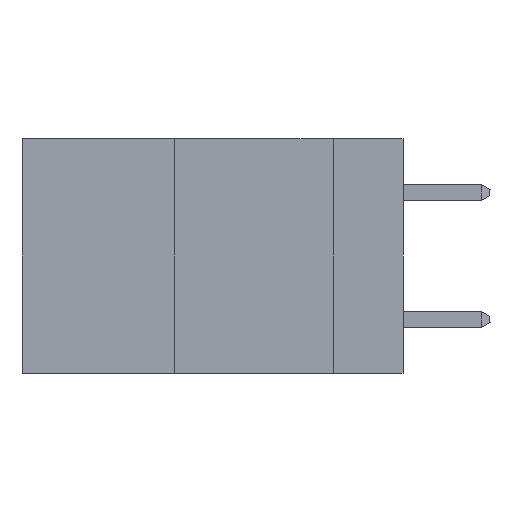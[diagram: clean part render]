
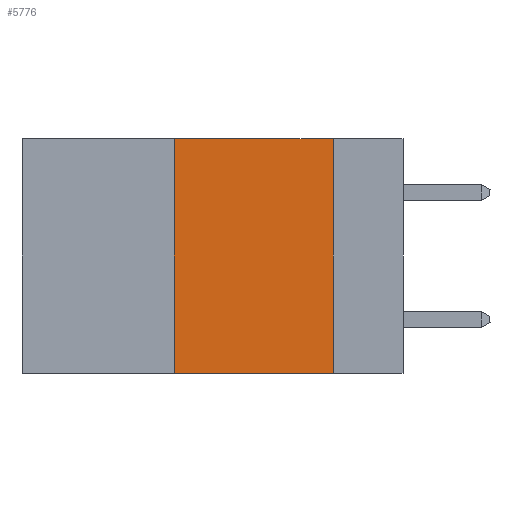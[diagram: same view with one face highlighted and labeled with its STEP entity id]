
A CAD part, left-side view. The second image highlights one B-rep face of the part: STEP entity #5776.
In plain terms, the highlighted planar face has unit normal (-1, 0, 0).
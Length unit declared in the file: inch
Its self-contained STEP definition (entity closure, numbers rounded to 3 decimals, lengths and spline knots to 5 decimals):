
#298 = DIRECTION ( 'NONE',  ( 0., 0., -1. ) ) ;
#560 = VECTOR ( 'NONE', #26376, 39.37008 ) ;
#3528 = CARTESIAN_POINT ( 'NONE',  ( 0., 0.11, 0. ) ) ;
#5776 = ADVANCED_FACE ( 'NONE', ( #25094 ), #15603, .F. ) ;
#8339 = VERTEX_POINT ( 'NONE', #15843 ) ;
#8670 = LINE ( 'NONE', #34059, #17646 ) ;
#11580 = VECTOR ( 'NONE', #31246, 39.37008 ) ;
#11921 = CARTESIAN_POINT ( 'NONE',  ( 0., 0.11, 0. ) ) ;
#13233 = VECTOR ( 'NONE', #298, 39.37008 ) ;
#13871 = DIRECTION ( 'NONE',  ( 0., -1., 0. ) ) ;
#14397 = LINE ( 'NONE', #29242, #560 ) ;
#15320 = ORIENTED_EDGE ( 'NONE', *, *, #20392, .T. ) ;
#15603 = PLANE ( 'NONE',  #24603 ) ;
#15730 = ORIENTED_EDGE ( 'NONE', *, *, #36065, .F. ) ;
#15843 = CARTESIAN_POINT ( 'NONE',  ( 0., 0.11, -0.37 ) ) ;
#17646 = VECTOR ( 'NONE', #13871, 39.37008 ) ;
#18300 = ORIENTED_EDGE ( 'NONE', *, *, #29711, .F. ) ;
#18983 = CARTESIAN_POINT ( 'NONE',  ( 0., 0.36, -0.37 ) ) ;
#19052 = EDGE_CURVE ( 'NONE', #30870, #8339, #20879, .T. ) ;
#19805 = CARTESIAN_POINT ( 'NONE',  ( 0., 0.36, 0. ) ) ;
#20392 = EDGE_CURVE ( 'NONE', #30541, #8339, #14397, .T. ) ;
#20879 = LINE ( 'NONE', #3528, #13233 ) ;
#22206 = ORIENTED_EDGE ( 'NONE', *, *, #19052, .F. ) ;
#22799 = VERTEX_POINT ( 'NONE', #34999 ) ;
#24312 = DIRECTION ( 'NONE',  ( 1., 0., 0. ) ) ;
#24603 = AXIS2_PLACEMENT_3D ( 'NONE', #27428, #24312, #35400 ) ;
#25052 = EDGE_LOOP ( 'NONE', ( #22206, #15730, #18300, #15320 ) ) ;
#25094 = FACE_OUTER_BOUND ( 'NONE', #25052, .T. ) ;
#26376 = DIRECTION ( 'NONE',  ( 0., -1., 0. ) ) ;
#27428 = CARTESIAN_POINT ( 'NONE',  ( 0., 0.6, 0. ) ) ;
#29242 = CARTESIAN_POINT ( 'NONE',  ( 0., 0.6, -0.37 ) ) ;
#29537 = LINE ( 'NONE', #19805, #11580 ) ;
#29711 = EDGE_CURVE ( 'NONE', #30541, #22799, #29537, .T. ) ;
#30541 = VERTEX_POINT ( 'NONE', #18983 ) ;
#30870 = VERTEX_POINT ( 'NONE', #11921 ) ;
#31246 = DIRECTION ( 'NONE',  ( 0., 0., 1. ) ) ;
#34059 = CARTESIAN_POINT ( 'NONE',  ( 0., 0.6, 0. ) ) ;
#34999 = CARTESIAN_POINT ( 'NONE',  ( 0., 0.36, 0. ) ) ;
#35400 = DIRECTION ( 'NONE',  ( 0., 0., -1. ) ) ;
#36065 = EDGE_CURVE ( 'NONE', #22799, #30870, #8670, .T. ) ;
